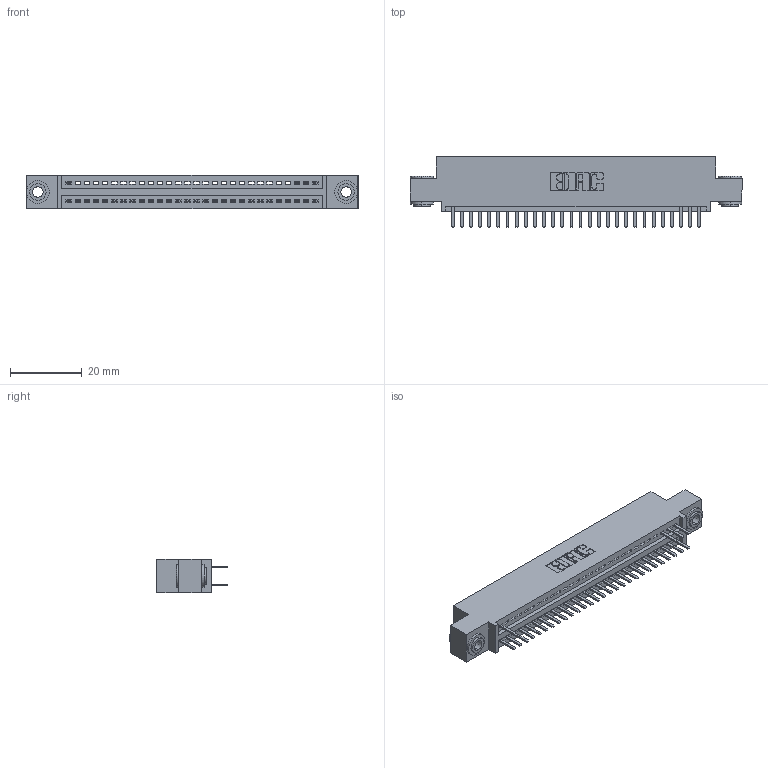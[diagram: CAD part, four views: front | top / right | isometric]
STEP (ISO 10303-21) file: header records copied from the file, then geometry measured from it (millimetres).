
FILE_DESCRIPTION (( 'STEP AP203' ), '1' );
FILE_NAME ('345-056-520-503.STEP', '2018-09-24T07:06:25', ( '' ), ( '' ), 'SwSTEP 2.0', 'SolidWorks 2016', '' );
FILE_SCHEMA (( 'CONFIG_CONTROL_DESIGN' ));
Length unit declared in the file: inch
Products named in the file (4): 345 Part_0.110 Offset - 0.156 Dia-TH; 345-292-001_345-293-120; 345-250-002_345-250-002-102; 345-056-520-503
Assembly tree (35 placements, depth 2):
  345-056-520-503
    345 Part_0.110 Offset - 0.156 Dia-TH
    345-292-001_345-293-120  x32
    345-250-002_345-250-002-102  x2
Bounding box: 92.33 x 19.68 x 9.4 mm (x, y, z)
Volume: 8554.6 mm3; surface area: 11416.5 mm2
Topology: 35 solids, 35 shells, 2088 faces, 6101 edges, 3978 vertices
Faces by surface type: plane 1382, cylinder 698, cone 8
Entity records: 23982 total; most frequent: CARTESIAN_POINT 4127, ORIENTED_EDGE 4066, DIRECTION 3647, EDGE_CURVE 2033, LINE 1761, VECTOR 1761, VERTEX_POINT 1350, AXIS2_PLACEMENT_3D 943
